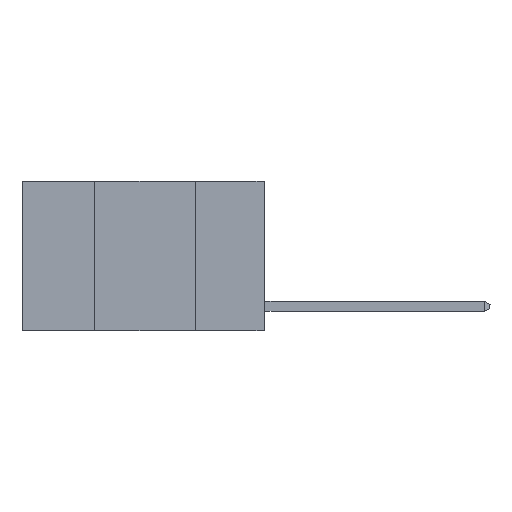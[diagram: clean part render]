
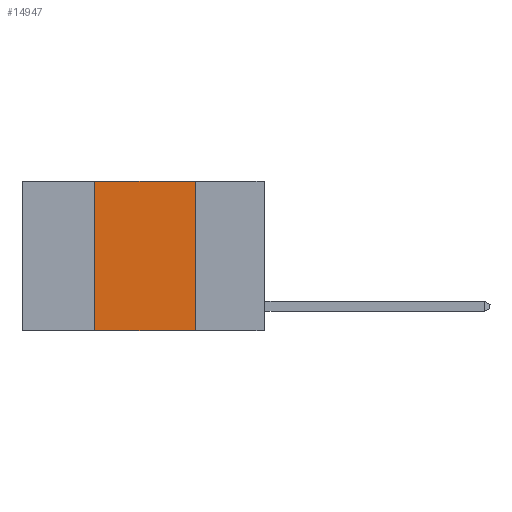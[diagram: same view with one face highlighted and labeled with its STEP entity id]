
A CAD part, left-side view. The second image highlights one B-rep face of the part: STEP entity #14947.
In plain terms, the highlighted planar face has unit normal (-1, 0, 0).
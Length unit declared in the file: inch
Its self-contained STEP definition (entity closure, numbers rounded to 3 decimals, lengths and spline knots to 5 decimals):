
#1841 = VECTOR ( 'NONE', #19673, 39.37008 ) ;
#2148 = LINE ( 'NONE', #15644, #13481 ) ;
#2765 = CARTESIAN_POINT ( 'NONE',  ( 0., 0.17, 0. ) ) ;
#3048 = FACE_OUTER_BOUND ( 'NONE', #22265, .T. ) ;
#3196 = ORIENTED_EDGE ( 'NONE', *, *, #22359, .T. ) ;
#3836 = LINE ( 'NONE', #2765, #1841 ) ;
#4218 = ORIENTED_EDGE ( 'NONE', *, *, #16844, .F. ) ;
#4452 = CARTESIAN_POINT ( 'NONE',  ( 0., 0.42, 0. ) ) ;
#4612 = ORIENTED_EDGE ( 'NONE', *, *, #7640, .F. ) ;
#4802 = VECTOR ( 'NONE', #14125, 39.37008 ) ;
#5295 = VERTEX_POINT ( 'NONE', #4452 ) ;
#5793 = DIRECTION ( 'NONE',  ( 0., -1., 0. ) ) ;
#6006 = CARTESIAN_POINT ( 'NONE',  ( 0., 0.17, -0.37 ) ) ;
#7640 = EDGE_CURVE ( 'NONE', #12839, #5295, #11111, .T. ) ;
#7650 = CARTESIAN_POINT ( 'NONE',  ( 0., 0.42, -0.37 ) ) ;
#9649 = LINE ( 'NONE', #18425, #26235 ) ;
#11111 = LINE ( 'NONE', #11990, #4802 ) ;
#11339 = DIRECTION ( 'NONE',  ( 1., 0., 0. ) ) ;
#11513 = DIRECTION ( 'NONE',  ( 0., -1., 0. ) ) ;
#11990 = CARTESIAN_POINT ( 'NONE',  ( 0., 0.42, 0. ) ) ;
#12839 = VERTEX_POINT ( 'NONE', #7650 ) ;
#13481 = VECTOR ( 'NONE', #11513, 39.37008 ) ;
#14125 = DIRECTION ( 'NONE',  ( 0., 0., 1. ) ) ;
#14947 = ADVANCED_FACE ( 'NONE', ( #3048 ), #23818, .F. ) ;
#15422 = ORIENTED_EDGE ( 'NONE', *, *, #21696, .F. ) ;
#15644 = CARTESIAN_POINT ( 'NONE',  ( 0., 0.6, -0.37 ) ) ;
#16319 = AXIS2_PLACEMENT_3D ( 'NONE', #17559, #11339, #25865 ) ;
#16385 = VERTEX_POINT ( 'NONE', #6006 ) ;
#16844 = EDGE_CURVE ( 'NONE', #5295, #20435, #9649, .T. ) ;
#17559 = CARTESIAN_POINT ( 'NONE',  ( 0., 0.6, 0. ) ) ;
#17618 = CARTESIAN_POINT ( 'NONE',  ( 0., 0.17, 0. ) ) ;
#18425 = CARTESIAN_POINT ( 'NONE',  ( 0., 0.6, 0. ) ) ;
#19673 = DIRECTION ( 'NONE',  ( 0., 0., -1. ) ) ;
#20435 = VERTEX_POINT ( 'NONE', #17618 ) ;
#21696 = EDGE_CURVE ( 'NONE', #20435, #16385, #3836, .T. ) ;
#22265 = EDGE_LOOP ( 'NONE', ( #15422, #4218, #4612, #3196 ) ) ;
#22359 = EDGE_CURVE ( 'NONE', #12839, #16385, #2148, .T. ) ;
#23818 = PLANE ( 'NONE',  #16319 ) ;
#25865 = DIRECTION ( 'NONE',  ( 0., 0., -1. ) ) ;
#26235 = VECTOR ( 'NONE', #5793, 39.37008 ) ;
